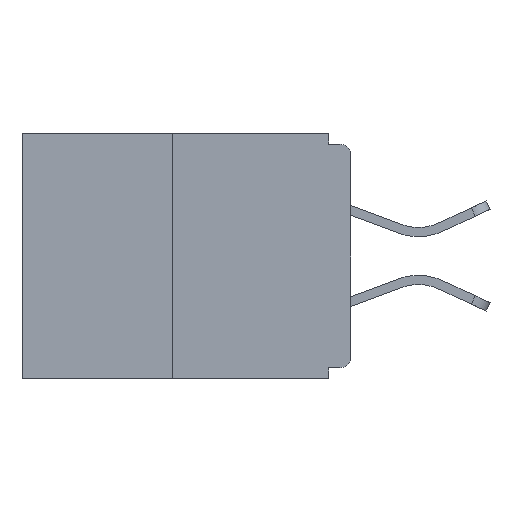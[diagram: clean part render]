
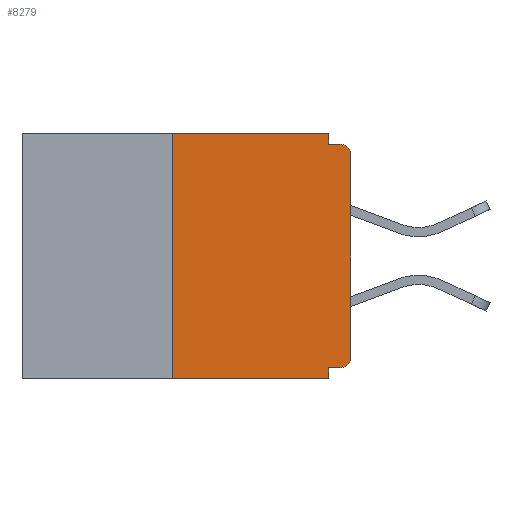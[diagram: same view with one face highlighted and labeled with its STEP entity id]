
A CAD part, left-side view. The second image highlights one B-rep face of the part: STEP entity #8279.
In plain terms, the highlighted planar face has unit normal (-1, 0, 0).
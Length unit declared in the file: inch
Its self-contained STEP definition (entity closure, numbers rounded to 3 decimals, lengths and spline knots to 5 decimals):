
#160 = ORIENTED_EDGE ( 'NONE', *, *, #4162, .T. ) ;
#244 = LINE ( 'NONE', #1128, #8780 ) ;
#396 = EDGE_CURVE ( 'NONE', #16584, #27552, #18804, .T. ) ;
#545 = ORIENTED_EDGE ( 'NONE', *, *, #1962, .F. ) ;
#1128 = CARTESIAN_POINT ( 'NONE',  ( 0., 0.46, 0. ) ) ;
#1198 = EDGE_CURVE ( 'NONE', #17643, #18206, #12379, .T. ) ;
#1669 = ORIENTED_EDGE ( 'NONE', *, *, #14339, .F. ) ;
#1962 = EDGE_CURVE ( 'NONE', #7242, #12995, #18521, .T. ) ;
#2108 = DIRECTION ( 'NONE',  ( 0., 0., -1. ) ) ;
#2483 = DIRECTION ( 'NONE',  ( 1., 0., 0. ) ) ;
#2904 = EDGE_CURVE ( 'NONE', #10830, #7242, #10955, .T. ) ;
#2907 = DIRECTION ( 'NONE',  ( 0., -1., 0. ) ) ;
#3059 = LINE ( 'NONE', #4951, #26589 ) ;
#3638 = DIRECTION ( 'NONE',  ( 0., 0., 1. ) ) ;
#3731 = CARTESIAN_POINT ( 'NONE',  ( 0., 0.25, 0. ) ) ;
#4034 = EDGE_LOOP ( 'NONE', ( #1669, #28405, #20171, #11600, #23633, #4608, #28460, #160, #545, #7001 ) ) ;
#4096 = CARTESIAN_POINT ( 'NONE',  ( 0., 0.25, -0.343 ) ) ;
#4162 = EDGE_CURVE ( 'NONE', #24698, #12995, #19107, .T. ) ;
#4608 = ORIENTED_EDGE ( 'NONE', *, *, #14139, .T. ) ;
#4924 = VECTOR ( 'NONE', #2108, 39.37008 ) ;
#4951 = CARTESIAN_POINT ( 'NONE',  ( 0., 0., 0. ) ) ;
#5467 = CARTESIAN_POINT ( 'NONE',  ( 0., 0.031, -0.343 ) ) ;
#5613 = CARTESIAN_POINT ( 'NONE',  ( 0., 0., -0.328 ) ) ;
#5674 = VECTOR ( 'NONE', #19047, 39.37008 ) ;
#5814 = DIRECTION ( 'NONE',  ( 0., 1., 0. ) ) ;
#7001 = ORIENTED_EDGE ( 'NONE', *, *, #2904, .F. ) ;
#7218 = VECTOR ( 'NONE', #5814, 39.37008 ) ;
#7224 = VERTEX_POINT ( 'NONE', #22058 ) ;
#7242 = VERTEX_POINT ( 'NONE', #19355 ) ;
#8178 = DIRECTION ( 'NONE',  ( 0., 0., -1. ) ) ;
#8279 = ADVANCED_FACE ( 'NONE', ( #16262 ), #20883, .F. ) ;
#8305 = LINE ( 'NONE', #5613, #7218 ) ;
#8408 = CARTESIAN_POINT ( 'NONE',  ( 0., 0.031, -0.343 ) ) ;
#8675 = CARTESIAN_POINT ( 'NONE',  ( 0., 0., -0.313 ) ) ;
#8780 = VECTOR ( 'NONE', #2907, 39.37008 ) ;
#9647 = CARTESIAN_POINT ( 'NONE',  ( 0., 0.031, 0. ) ) ;
#10830 = VERTEX_POINT ( 'NONE', #9647 ) ;
#10870 = AXIS2_PLACEMENT_3D ( 'NONE', #24365, #17365, #8178 ) ;
#10928 = VECTOR ( 'NONE', #3638, 39.37008 ) ;
#10955 = LINE ( 'NONE', #18102, #4924 ) ;
#11600 = ORIENTED_EDGE ( 'NONE', *, *, #396, .F. ) ;
#11679 = CARTESIAN_POINT ( 'NONE',  ( 0., 0.015, -0.03 ) ) ;
#11693 = LINE ( 'NONE', #26058, #5674 ) ;
#12379 = LINE ( 'NONE', #3731, #10928 ) ;
#12995 = VERTEX_POINT ( 'NONE', #16473 ) ;
#14124 = DIRECTION ( 'NONE',  ( 0., 0., -1. ) ) ;
#14139 = EDGE_CURVE ( 'NONE', #7224, #26501, #28385, .T. ) ;
#14339 = EDGE_CURVE ( 'NONE', #18206, #10830, #244, .T. ) ;
#16262 = FACE_OUTER_BOUND ( 'NONE', #4034, .T. ) ;
#16473 = CARTESIAN_POINT ( 'NONE',  ( 0., 0.015, -0.015 ) ) ;
#16584 = VERTEX_POINT ( 'NONE', #28770 ) ;
#17365 = DIRECTION ( 'NONE',  ( -1., 0., 0. ) ) ;
#17643 = VERTEX_POINT ( 'NONE', #4096 ) ;
#18102 = CARTESIAN_POINT ( 'NONE',  ( 0., 0.031, 0. ) ) ;
#18206 = VERTEX_POINT ( 'NONE', #21109 ) ;
#18521 = LINE ( 'NONE', #21145, #22481 ) ;
#18804 = LINE ( 'NONE', #8408, #22747 ) ;
#19047 = DIRECTION ( 'NONE',  ( 0., -1., 0. ) ) ;
#19107 = CIRCLE ( 'NONE', #27548, 0.015 ) ;
#19355 = CARTESIAN_POINT ( 'NONE',  ( 0., 0.031, -0.015 ) ) ;
#20171 = ORIENTED_EDGE ( 'NONE', *, *, #21312, .T. ) ;
#20846 = DIRECTION ( 'NONE',  ( -1., 0., 0. ) ) ;
#20873 = DIRECTION ( 'NONE',  ( 0., 0., 1. ) ) ;
#20883 = PLANE ( 'NONE',  #26870 ) ;
#21109 = CARTESIAN_POINT ( 'NONE',  ( 0., 0.25, 0. ) ) ;
#21145 = CARTESIAN_POINT ( 'NONE',  ( 0., 0., -0.015 ) ) ;
#21312 = EDGE_CURVE ( 'NONE', #17643, #27552, #11693, .T. ) ;
#22058 = CARTESIAN_POINT ( 'NONE',  ( 0., 0.015, -0.328 ) ) ;
#22481 = VECTOR ( 'NONE', #23344, 39.37008 ) ;
#22747 = VECTOR ( 'NONE', #24406, 39.37008 ) ;
#22957 = DIRECTION ( 'NONE',  ( 0., 0., -1. ) ) ;
#23344 = DIRECTION ( 'NONE',  ( 0., -1., 0. ) ) ;
#23468 = EDGE_CURVE ( 'NONE', #26501, #24698, #3059, .T. ) ;
#23633 = ORIENTED_EDGE ( 'NONE', *, *, #29383, .F. ) ;
#24365 = CARTESIAN_POINT ( 'NONE',  ( 0., 0.015, -0.313 ) ) ;
#24406 = DIRECTION ( 'NONE',  ( 0., 0., -1. ) ) ;
#24698 = VERTEX_POINT ( 'NONE', #25807 ) ;
#25504 = CARTESIAN_POINT ( 'NONE',  ( 0., 0.46, 0. ) ) ;
#25807 = CARTESIAN_POINT ( 'NONE',  ( 0., 0., -0.03 ) ) ;
#26058 = CARTESIAN_POINT ( 'NONE',  ( 0., 0.46, -0.343 ) ) ;
#26501 = VERTEX_POINT ( 'NONE', #8675 ) ;
#26589 = VECTOR ( 'NONE', #20873, 39.37008 ) ;
#26870 = AXIS2_PLACEMENT_3D ( 'NONE', #25504, #2483, #14124 ) ;
#27548 = AXIS2_PLACEMENT_3D ( 'NONE', #11679, #20846, #22957 ) ;
#27552 = VERTEX_POINT ( 'NONE', #5467 ) ;
#28385 = CIRCLE ( 'NONE', #10870, 0.015 ) ;
#28405 = ORIENTED_EDGE ( 'NONE', *, *, #1198, .F. ) ;
#28460 = ORIENTED_EDGE ( 'NONE', *, *, #23468, .T. ) ;
#28770 = CARTESIAN_POINT ( 'NONE',  ( 0., 0.031, -0.328 ) ) ;
#29383 = EDGE_CURVE ( 'NONE', #7224, #16584, #8305, .T. ) ;
